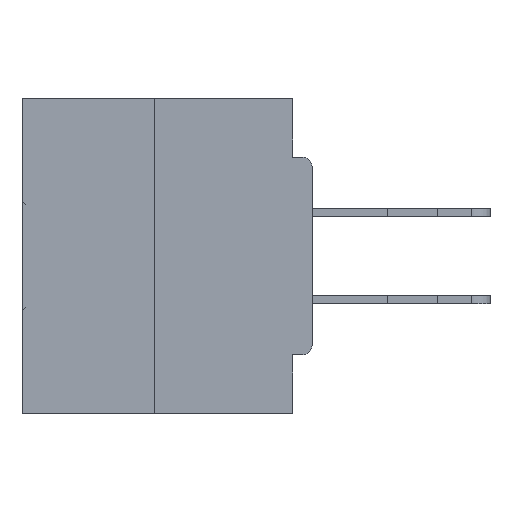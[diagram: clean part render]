
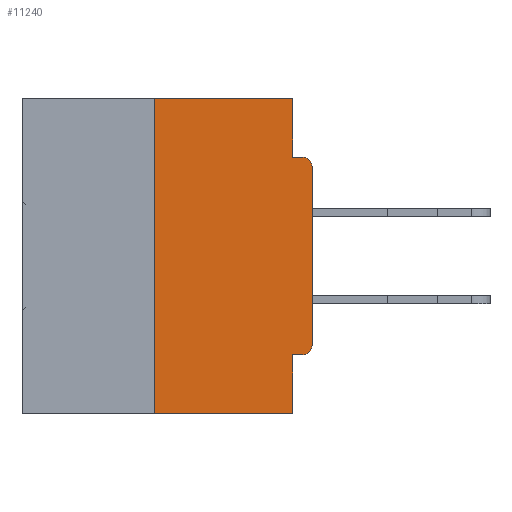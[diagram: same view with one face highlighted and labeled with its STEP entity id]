
A CAD part, left-side view. The second image highlights one B-rep face of the part: STEP entity #11240.
In plain terms, the highlighted planar face has unit normal (-1, 0, 0).
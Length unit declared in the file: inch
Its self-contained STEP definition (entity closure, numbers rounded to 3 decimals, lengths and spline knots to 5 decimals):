
#475 = VERTEX_POINT ( 'NONE', #16692 ) ;
#572 = CARTESIAN_POINT ( 'NONE',  ( 0., 0.031, 0. ) ) ;
#720 = PLANE ( 'NONE',  #21487 ) ;
#808 = LINE ( 'NONE', #19745, #12406 ) ;
#989 = DIRECTION ( 'NONE',  ( -1., 0., 0. ) ) ;
#1235 = ORIENTED_EDGE ( 'NONE', *, *, #30278, .T. ) ;
#1293 = CARTESIAN_POINT ( 'NONE',  ( 0., 0.015, -0.1085 ) ) ;
#2127 = VECTOR ( 'NONE', #18547, 39.37008 ) ;
#2144 = AXIS2_PLACEMENT_3D ( 'NONE', #1293, #989, #22611 ) ;
#2689 = CARTESIAN_POINT ( 'NONE',  ( 0., 0., -0.0935 ) ) ;
#3887 = ORIENTED_EDGE ( 'NONE', *, *, #44518, .T. ) ;
#4103 = CARTESIAN_POINT ( 'NONE',  ( 0., 0.46, 0. ) ) ;
#4220 = LINE ( 'NONE', #18002, #6413 ) ;
#4259 = DIRECTION ( 'NONE',  ( 1., 0., 0. ) ) ;
#5883 = CARTESIAN_POINT ( 'NONE',  ( 0., 0.25, 0. ) ) ;
#6413 = VECTOR ( 'NONE', #42638, 39.37008 ) ;
#7019 = VERTEX_POINT ( 'NONE', #27925 ) ;
#7511 = CARTESIAN_POINT ( 'NONE',  ( 0., 0.25, 0. ) ) ;
#7745 = CARTESIAN_POINT ( 'NONE',  ( 0., 0.031, -0.0935 ) ) ;
#8776 = LINE ( 'NONE', #25643, #26423 ) ;
#9490 = DIRECTION ( 'NONE',  ( 0., -1., 0. ) ) ;
#10401 = EDGE_CURVE ( 'NONE', #45652, #37087, #808, .T. ) ;
#10428 = CARTESIAN_POINT ( 'NONE',  ( 0., 0.25, -0.5 ) ) ;
#10955 = CARTESIAN_POINT ( 'NONE',  ( 0., 0.46, 0. ) ) ;
#11240 = ADVANCED_FACE ( 'NONE', ( #29421 ), #720, .F. ) ;
#11256 = VERTEX_POINT ( 'NONE', #572 ) ;
#11574 = ORIENTED_EDGE ( 'NONE', *, *, #21611, .F. ) ;
#12147 = VECTOR ( 'NONE', #31979, 39.37008 ) ;
#12406 = VECTOR ( 'NONE', #31888, 39.37008 ) ;
#12659 = CIRCLE ( 'NONE', #15675, 0.015 ) ;
#12876 = ORIENTED_EDGE ( 'NONE', *, *, #13336, .F. ) ;
#12995 = EDGE_CURVE ( 'NONE', #38588, #475, #20943, .T. ) ;
#13336 = EDGE_CURVE ( 'NONE', #11256, #38588, #8776, .T. ) ;
#14560 = CARTESIAN_POINT ( 'NONE',  ( 0., 0.031, -0.4065 ) ) ;
#15356 = EDGE_CURVE ( 'NONE', #39227, #30207, #4220, .T. ) ;
#15675 = AXIS2_PLACEMENT_3D ( 'NONE', #33817, #20250, #23235 ) ;
#15791 = CARTESIAN_POINT ( 'NONE',  ( 0., 0.031, -0.5 ) ) ;
#16692 = CARTESIAN_POINT ( 'NONE',  ( 0., 0.015, -0.0935 ) ) ;
#17718 = CARTESIAN_POINT ( 'NONE',  ( 0., 0.015, -0.4065 ) ) ;
#18002 = CARTESIAN_POINT ( 'NONE',  ( 0., 0., -0.4065 ) ) ;
#18547 = DIRECTION ( 'NONE',  ( 0., 0., 1. ) ) ;
#19745 = CARTESIAN_POINT ( 'NONE',  ( 0., 0.46, -0.5 ) ) ;
#20250 = DIRECTION ( 'NONE',  ( -1., 0., 0. ) ) ;
#20943 = LINE ( 'NONE', #2689, #23176 ) ;
#21487 = AXIS2_PLACEMENT_3D ( 'NONE', #4103, #4259, #29124 ) ;
#21611 = EDGE_CURVE ( 'NONE', #45652, #24832, #37495, .T. ) ;
#21754 = DIRECTION ( 'NONE',  ( 0., 0., -1. ) ) ;
#22611 = DIRECTION ( 'NONE',  ( 0., 0., -1. ) ) ;
#23176 = VECTOR ( 'NONE', #9490, 39.37008 ) ;
#23208 = ORIENTED_EDGE ( 'NONE', *, *, #25701, .F. ) ;
#23235 = DIRECTION ( 'NONE',  ( 0., 0., -1. ) ) ;
#24832 = VERTEX_POINT ( 'NONE', #5883 ) ;
#25163 = CARTESIAN_POINT ( 'NONE',  ( 0., 0.031, -0.5 ) ) ;
#25643 = CARTESIAN_POINT ( 'NONE',  ( 0., 0.031, 0. ) ) ;
#25701 = EDGE_CURVE ( 'NONE', #30207, #37087, #29836, .T. ) ;
#26017 = CARTESIAN_POINT ( 'NONE',  ( 0., 0., -0.3915 ) ) ;
#26183 = ORIENTED_EDGE ( 'NONE', *, *, #10401, .T. ) ;
#26423 = VECTOR ( 'NONE', #35960, 39.37008 ) ;
#27623 = EDGE_LOOP ( 'NONE', ( #37864, #11574, #26183, #23208, #36891, #3887, #1235, #34410, #38659, #12876 ) ) ;
#27628 = CIRCLE ( 'NONE', #2144, 0.015 ) ;
#27925 = CARTESIAN_POINT ( 'NONE',  ( 0., 0., -0.1085 ) ) ;
#28863 = DIRECTION ( 'NONE',  ( 0., -1., 0. ) ) ;
#29124 = DIRECTION ( 'NONE',  ( 0., 0., -1. ) ) ;
#29175 = EDGE_CURVE ( 'NONE', #7019, #475, #27628, .T. ) ;
#29421 = FACE_OUTER_BOUND ( 'NONE', #27623, .T. ) ;
#29813 = LINE ( 'NONE', #10955, #44692 ) ;
#29836 = LINE ( 'NONE', #25163, #32018 ) ;
#30207 = VERTEX_POINT ( 'NONE', #14560 ) ;
#30278 = EDGE_CURVE ( 'NONE', #35693, #7019, #43548, .T. ) ;
#31888 = DIRECTION ( 'NONE',  ( 0., -1., 0. ) ) ;
#31979 = DIRECTION ( 'NONE',  ( 0., 0., 1. ) ) ;
#32018 = VECTOR ( 'NONE', #21754, 39.37008 ) ;
#33817 = CARTESIAN_POINT ( 'NONE',  ( 0., 0.015, -0.3915 ) ) ;
#34410 = ORIENTED_EDGE ( 'NONE', *, *, #29175, .T. ) ;
#35693 = VERTEX_POINT ( 'NONE', #26017 ) ;
#35960 = DIRECTION ( 'NONE',  ( 0., 0., -1. ) ) ;
#36891 = ORIENTED_EDGE ( 'NONE', *, *, #15356, .F. ) ;
#37087 = VERTEX_POINT ( 'NONE', #15791 ) ;
#37495 = LINE ( 'NONE', #7511, #12147 ) ;
#37864 = ORIENTED_EDGE ( 'NONE', *, *, #40509, .F. ) ;
#38588 = VERTEX_POINT ( 'NONE', #7745 ) ;
#38659 = ORIENTED_EDGE ( 'NONE', *, *, #12995, .F. ) ;
#39227 = VERTEX_POINT ( 'NONE', #17718 ) ;
#40509 = EDGE_CURVE ( 'NONE', #24832, #11256, #29813, .T. ) ;
#42638 = DIRECTION ( 'NONE',  ( 0., 1., 0. ) ) ;
#43027 = CARTESIAN_POINT ( 'NONE',  ( 0., 0., 0. ) ) ;
#43548 = LINE ( 'NONE', #43027, #2127 ) ;
#44518 = EDGE_CURVE ( 'NONE', #39227, #35693, #12659, .T. ) ;
#44692 = VECTOR ( 'NONE', #28863, 39.37008 ) ;
#45652 = VERTEX_POINT ( 'NONE', #10428 ) ;
